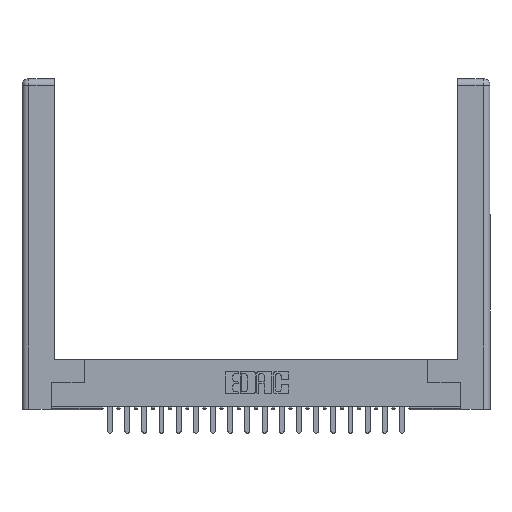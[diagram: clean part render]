
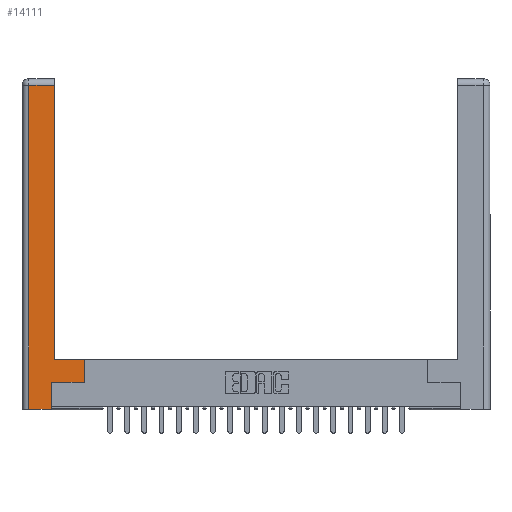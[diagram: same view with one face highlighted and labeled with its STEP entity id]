
A CAD part, top view. The second image highlights one B-rep face of the part: STEP entity #14111.
In plain terms, the highlighted planar face has unit normal (0, 0, 1).
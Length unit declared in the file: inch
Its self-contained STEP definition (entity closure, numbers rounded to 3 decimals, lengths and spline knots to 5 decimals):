
#27 = PLANE ( 'NONE',  #354 ) ;
#48 = VERTEX_POINT ( 'NONE', #22830 ) ;
#354 = AXIS2_PLACEMENT_3D ( 'NONE', #1723, #23147, #17171 ) ;
#809 = VECTOR ( 'NONE', #8289, 39.37008 ) ;
#982 = CARTESIAN_POINT ( 'NONE',  ( 0.265, 0.245, 0. ) ) ;
#1399 = ORIENTED_EDGE ( 'NONE', *, *, #19615, .T. ) ;
#1503 = LINE ( 'NONE', #9642, #9638 ) ;
#1723 = CARTESIAN_POINT ( 'NONE',  ( 0., 0., 0. ) ) ;
#2250 = CARTESIAN_POINT ( 'NONE',  ( 0.0615, 0., 0. ) ) ;
#2476 = VERTEX_POINT ( 'NONE', #23945 ) ;
#3672 = ORIENTED_EDGE ( 'NONE', *, *, #15315, .T. ) ;
#3731 = DIRECTION ( 'NONE',  ( 0., -1., 0. ) ) ;
#4368 = CARTESIAN_POINT ( 'NONE',  ( 0.265, 0., 0. ) ) ;
#4723 = VERTEX_POINT ( 'NONE', #2250 ) ;
#5177 = CARTESIAN_POINT ( 'NONE',  ( 0.0615, 2.94, 0. ) ) ;
#5505 = FACE_OUTER_BOUND ( 'NONE', #22311, .T. ) ;
#6017 = CARTESIAN_POINT ( 'NONE',  ( 0.565, 0.45, 0. ) ) ;
#6555 = VERTEX_POINT ( 'NONE', #19130 ) ;
#8003 = LINE ( 'NONE', #17361, #21523 ) ;
#8289 = DIRECTION ( 'NONE',  ( 1., 0., 0. ) ) ;
#8392 = EDGE_CURVE ( 'NONE', #14109, #11011, #1503, .T. ) ;
#8661 = LINE ( 'NONE', #5177, #23415 ) ;
#8724 = ORIENTED_EDGE ( 'NONE', *, *, #8392, .T. ) ;
#9638 = VECTOR ( 'NONE', #22922, 39.37008 ) ;
#9642 = CARTESIAN_POINT ( 'NONE',  ( 0.295, 0.45, 0. ) ) ;
#10108 = EDGE_CURVE ( 'NONE', #4723, #13309, #10137, .T. ) ;
#10137 = LINE ( 'NONE', #4368, #809 ) ;
#10231 = ORIENTED_EDGE ( 'NONE', *, *, #10331, .T. ) ;
#10331 = EDGE_CURVE ( 'NONE', #16220, #2476, #17363, .T. ) ;
#11011 = VERTEX_POINT ( 'NONE', #21897 ) ;
#11841 = LINE ( 'NONE', #6017, #19362 ) ;
#12246 = VECTOR ( 'NONE', #20886, 39.37008 ) ;
#12584 = LINE ( 'NONE', #17088, #22826 ) ;
#13115 = CARTESIAN_POINT ( 'NONE',  ( 0.565, 0.245, 0. ) ) ;
#13309 = VERTEX_POINT ( 'NONE', #22167 ) ;
#14109 = VERTEX_POINT ( 'NONE', #21055 ) ;
#14111 = ADVANCED_FACE ( 'NONE', ( #5505 ), #27, .F. ) ;
#15315 = EDGE_CURVE ( 'NONE', #6555, #4723, #12584, .T. ) ;
#16077 = DIRECTION ( 'NONE',  ( 0., 1., 0. ) ) ;
#16220 = VERTEX_POINT ( 'NONE', #982 ) ;
#17088 = CARTESIAN_POINT ( 'NONE',  ( 0.0615, 0., 0. ) ) ;
#17171 = DIRECTION ( 'NONE',  ( -1., 0., 0. ) ) ;
#17337 = DIRECTION ( 'NONE',  ( 0., 1., 0. ) ) ;
#17361 = CARTESIAN_POINT ( 'NONE',  ( 0.295, 3., 0. ) ) ;
#17363 = LINE ( 'NONE', #13115, #12246 ) ;
#18445 = EDGE_CURVE ( 'NONE', #11011, #48, #8003, .T. ) ;
#19130 = CARTESIAN_POINT ( 'NONE',  ( 0.0615, 2.94, 0. ) ) ;
#19362 = VECTOR ( 'NONE', #24292, 39.37008 ) ;
#19364 = CARTESIAN_POINT ( 'NONE',  ( 0.265, 0.245, 0. ) ) ;
#19615 = EDGE_CURVE ( 'NONE', #13309, #16220, #21045, .T. ) ;
#20426 = DIRECTION ( 'NONE',  ( -1., 0., 0. ) ) ;
#20545 = ORIENTED_EDGE ( 'NONE', *, *, #10108, .T. ) ;
#20561 = EDGE_CURVE ( 'NONE', #48, #6555, #8661, .T. ) ;
#20886 = DIRECTION ( 'NONE',  ( 1., 0., 0. ) ) ;
#21045 = LINE ( 'NONE', #19364, #22222 ) ;
#21055 = CARTESIAN_POINT ( 'NONE',  ( 0.565, 0.45, 0. ) ) ;
#21523 = VECTOR ( 'NONE', #16077, 39.37008 ) ;
#21897 = CARTESIAN_POINT ( 'NONE',  ( 0.295, 0.45, 0. ) ) ;
#22167 = CARTESIAN_POINT ( 'NONE',  ( 0.265, 0., 0. ) ) ;
#22171 = ORIENTED_EDGE ( 'NONE', *, *, #18445, .T. ) ;
#22222 = VECTOR ( 'NONE', #17337, 39.37008 ) ;
#22311 = EDGE_LOOP ( 'NONE', ( #22171, #22526, #3672, #20545, #1399, #10231, #23775, #8724 ) ) ;
#22526 = ORIENTED_EDGE ( 'NONE', *, *, #20561, .T. ) ;
#22826 = VECTOR ( 'NONE', #3731, 39.37008 ) ;
#22830 = CARTESIAN_POINT ( 'NONE',  ( 0.295, 2.94, 0. ) ) ;
#22922 = DIRECTION ( 'NONE',  ( -1., 0., 0. ) ) ;
#23147 = DIRECTION ( 'NONE',  ( 0., 0., -1. ) ) ;
#23160 = EDGE_CURVE ( 'NONE', #2476, #14109, #11841, .T. ) ;
#23415 = VECTOR ( 'NONE', #20426, 39.37008 ) ;
#23775 = ORIENTED_EDGE ( 'NONE', *, *, #23160, .T. ) ;
#23945 = CARTESIAN_POINT ( 'NONE',  ( 0.565, 0.245, 0. ) ) ;
#24292 = DIRECTION ( 'NONE',  ( 0., 1., 0. ) ) ;
